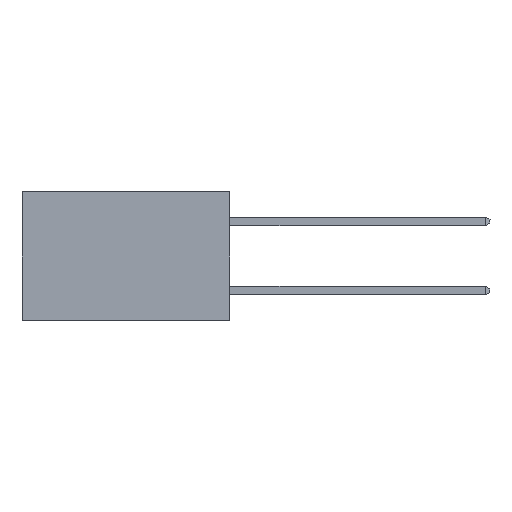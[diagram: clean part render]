
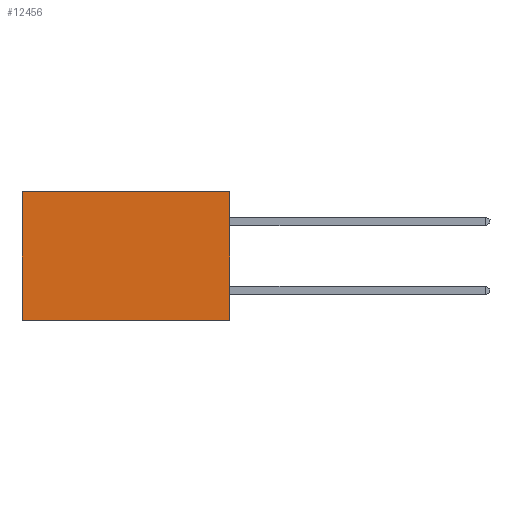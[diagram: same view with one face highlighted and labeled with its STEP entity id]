
A CAD part, left-side view. The second image highlights one B-rep face of the part: STEP entity #12456.
In plain terms, the highlighted planar face has unit normal (-1, 0, 0).
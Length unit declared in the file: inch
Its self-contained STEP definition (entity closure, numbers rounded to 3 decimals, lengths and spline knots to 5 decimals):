
#140 = CARTESIAN_POINT ( 'NONE',  ( 0.2615, 0., 0. ) ) ;
#153 = DIRECTION ( 'NONE',  ( 0., 0., -1. ) ) ;
#1155 = ORIENTED_EDGE ( 'NONE', *, *, #5584, .T. ) ;
#1175 = LINE ( 'NONE', #9917, #5619 ) ;
#1699 = CARTESIAN_POINT ( 'NONE',  ( 0.2615, 0.6, 0. ) ) ;
#2330 = PLANE ( 'NONE',  #2956 ) ;
#2535 = DIRECTION ( 'NONE',  ( 0., 0., -1. ) ) ;
#2707 = LINE ( 'NONE', #9936, #7678 ) ;
#2956 = AXIS2_PLACEMENT_3D ( 'NONE', #7431, #6267, #2535 ) ;
#3833 = EDGE_CURVE ( 'NONE', #8603, #7333, #2707, .T. ) ;
#3990 = ORIENTED_EDGE ( 'NONE', *, *, #3833, .T. ) ;
#4092 = DIRECTION ( 'NONE',  ( 0., 1., 0. ) ) ;
#5270 = CARTESIAN_POINT ( 'NONE',  ( 0.2615, 0., -0.37 ) ) ;
#5473 = ORIENTED_EDGE ( 'NONE', *, *, #8660, .F. ) ;
#5584 = EDGE_CURVE ( 'NONE', #6605, #8603, #5994, .T. ) ;
#5619 = VECTOR ( 'NONE', #4092, 39.37008 ) ;
#5994 = LINE ( 'NONE', #7814, #10887 ) ;
#6036 = CARTESIAN_POINT ( 'NONE',  ( 0.2615, 0., -0.37 ) ) ;
#6267 = DIRECTION ( 'NONE',  ( 1., 0., 0. ) ) ;
#6605 = VERTEX_POINT ( 'NONE', #140 ) ;
#7181 = VECTOR ( 'NONE', #9052, 39.37008 ) ;
#7232 = FACE_OUTER_BOUND ( 'NONE', #9022, .T. ) ;
#7333 = VERTEX_POINT ( 'NONE', #8757 ) ;
#7431 = CARTESIAN_POINT ( 'NONE',  ( 0.2615, 0., -0.37 ) ) ;
#7678 = VECTOR ( 'NONE', #153, 39.37008 ) ;
#7814 = CARTESIAN_POINT ( 'NONE',  ( 0.2615, 0., 0. ) ) ;
#8603 = VERTEX_POINT ( 'NONE', #1699 ) ;
#8660 = EDGE_CURVE ( 'NONE', #6605, #11258, #11879, .T. ) ;
#8757 = CARTESIAN_POINT ( 'NONE',  ( 0.2615, 0.6, -0.37 ) ) ;
#9022 = EDGE_LOOP ( 'NONE', ( #3990, #11673, #5473, #1155 ) ) ;
#9052 = DIRECTION ( 'NONE',  ( 0., 0., -1. ) ) ;
#9917 = CARTESIAN_POINT ( 'NONE',  ( 0.2615, 0., -0.37 ) ) ;
#9936 = CARTESIAN_POINT ( 'NONE',  ( 0.2615, 0.6, -0.37 ) ) ;
#10887 = VECTOR ( 'NONE', #11825, 39.37008 ) ;
#11258 = VERTEX_POINT ( 'NONE', #6036 ) ;
#11673 = ORIENTED_EDGE ( 'NONE', *, *, #11749, .F. ) ;
#11749 = EDGE_CURVE ( 'NONE', #11258, #7333, #1175, .T. ) ;
#11825 = DIRECTION ( 'NONE',  ( 0., 1., 0. ) ) ;
#11879 = LINE ( 'NONE', #5270, #7181 ) ;
#12456 = ADVANCED_FACE ( 'NONE', ( #7232 ), #2330, .F. ) ;
